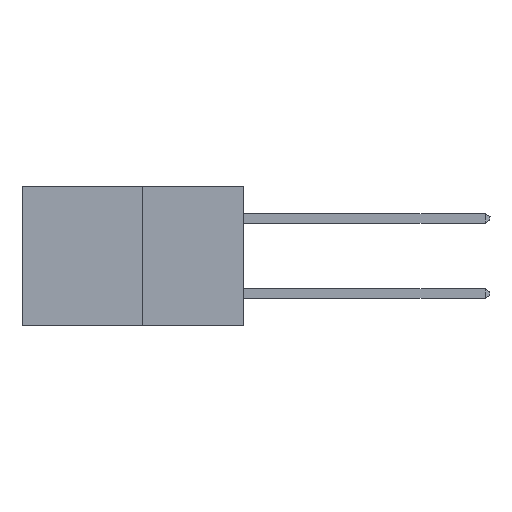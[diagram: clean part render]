
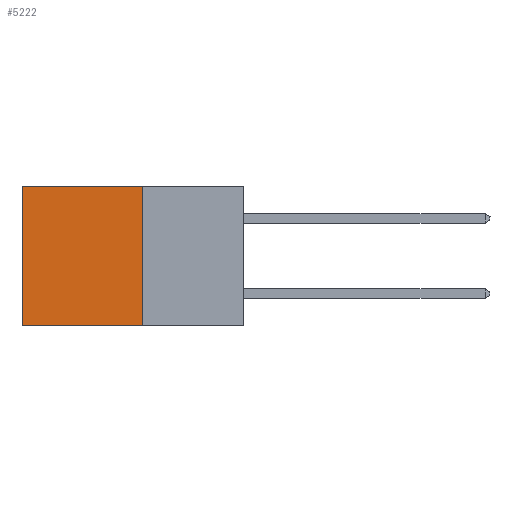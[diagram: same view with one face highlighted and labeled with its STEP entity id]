
A CAD part, left-side view. The second image highlights one B-rep face of the part: STEP entity #5222.
In plain terms, the highlighted planar face has unit normal (-1, 0, 0).
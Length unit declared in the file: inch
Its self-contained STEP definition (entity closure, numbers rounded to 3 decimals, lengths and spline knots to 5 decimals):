
#415 = VECTOR ( 'NONE', #15022, 39.37008 ) ;
#2200 = DIRECTION ( 'NONE',  ( 1., 0., 0. ) ) ;
#2965 = EDGE_CURVE ( 'NONE', #3117, #17589, #19299, .T. ) ;
#3117 = VERTEX_POINT ( 'NONE', #6136 ) ;
#4020 = DIRECTION ( 'NONE',  ( 0., 1., 0. ) ) ;
#5222 = ADVANCED_FACE ( 'NONE', ( #19038 ), #10439, .F. ) ;
#6136 = CARTESIAN_POINT ( 'NONE',  ( 0.277, 0.27, 0. ) ) ;
#6426 = CARTESIAN_POINT ( 'NONE',  ( 0.277, 0.27, -0.37 ) ) ;
#7132 = AXIS2_PLACEMENT_3D ( 'NONE', #12073, #2200, #13727 ) ;
#7221 = EDGE_CURVE ( 'NONE', #3117, #13437, #9696, .T. ) ;
#7754 = DIRECTION ( 'NONE',  ( 0., 0., -1. ) ) ;
#9472 = EDGE_CURVE ( 'NONE', #17589, #15803, #20884, .T. ) ;
#9696 = LINE ( 'NONE', #14941, #415 ) ;
#9851 = CARTESIAN_POINT ( 'NONE',  ( 0.277, 0.27, -0.37 ) ) ;
#9861 = EDGE_LOOP ( 'NONE', ( #15243, #18310, #18604, #16080 ) ) ;
#10382 = EDGE_CURVE ( 'NONE', #13437, #15803, #19530, .T. ) ;
#10439 = PLANE ( 'NONE',  #7132 ) ;
#11055 = CARTESIAN_POINT ( 'NONE',  ( 0.277, 0.59, -0.37 ) ) ;
#11208 = CARTESIAN_POINT ( 'NONE',  ( 0.277, 0.59, 0. ) ) ;
#11789 = CARTESIAN_POINT ( 'NONE',  ( 0.277, 0.59, -0.37 ) ) ;
#12073 = CARTESIAN_POINT ( 'NONE',  ( 0.277, 0.27, -0.37 ) ) ;
#13437 = VERTEX_POINT ( 'NONE', #11208 ) ;
#13577 = DIRECTION ( 'NONE',  ( 0., 0., -1. ) ) ;
#13727 = DIRECTION ( 'NONE',  ( 0., 0., -1. ) ) ;
#14472 = VECTOR ( 'NONE', #13577, 39.37008 ) ;
#14941 = CARTESIAN_POINT ( 'NONE',  ( 0.277, 0.27, 0. ) ) ;
#15022 = DIRECTION ( 'NONE',  ( 0., 1., 0. ) ) ;
#15243 = ORIENTED_EDGE ( 'NONE', *, *, #10382, .T. ) ;
#15803 = VERTEX_POINT ( 'NONE', #11789 ) ;
#16080 = ORIENTED_EDGE ( 'NONE', *, *, #7221, .T. ) ;
#16555 = VECTOR ( 'NONE', #4020, 39.37008 ) ;
#17589 = VERTEX_POINT ( 'NONE', #9851 ) ;
#18310 = ORIENTED_EDGE ( 'NONE', *, *, #9472, .F. ) ;
#18604 = ORIENTED_EDGE ( 'NONE', *, *, #2965, .F. ) ;
#19020 = VECTOR ( 'NONE', #7754, 39.37008 ) ;
#19038 = FACE_OUTER_BOUND ( 'NONE', #9861, .T. ) ;
#19299 = LINE ( 'NONE', #6426, #14472 ) ;
#19530 = LINE ( 'NONE', #11055, #19020 ) ;
#20366 = CARTESIAN_POINT ( 'NONE',  ( 0.277, 0.27, -0.37 ) ) ;
#20884 = LINE ( 'NONE', #20366, #16555 ) ;
